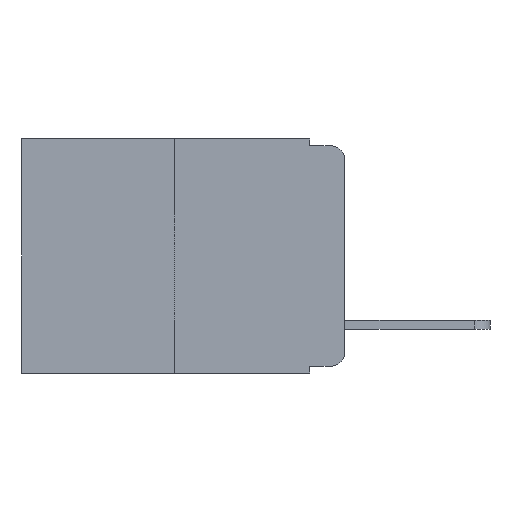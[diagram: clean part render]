
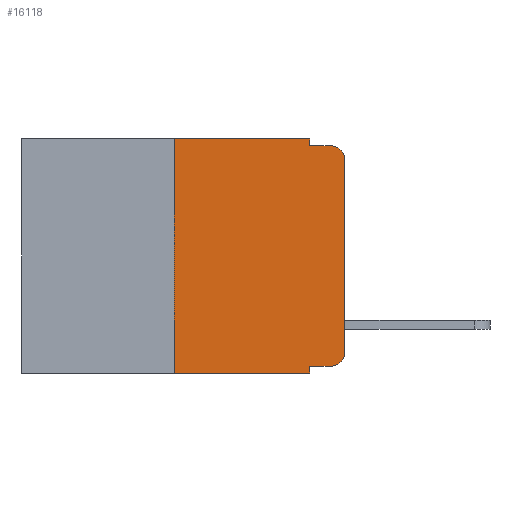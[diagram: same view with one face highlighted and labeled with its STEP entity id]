
A CAD part, left-side view. The second image highlights one B-rep face of the part: STEP entity #16118.
In plain terms, the highlighted planar face has unit normal (-1, 0, 0).
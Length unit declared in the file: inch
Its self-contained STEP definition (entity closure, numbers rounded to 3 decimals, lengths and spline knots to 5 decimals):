
#192 = ORIENTED_EDGE ( 'NONE', *, *, #7527, .T. ) ;
#748 = CARTESIAN_POINT ( 'NONE',  ( 0., 0.051, 0. ) ) ;
#917 = VERTEX_POINT ( 'NONE', #7803 ) ;
#1112 = CARTESIAN_POINT ( 'NONE',  ( 0., 0.02, -0.01 ) ) ;
#1442 = CARTESIAN_POINT ( 'NONE',  ( 0., 0.051, -0.343 ) ) ;
#1617 = DIRECTION ( 'NONE',  ( 0., 0., -1. ) ) ;
#1857 = ORIENTED_EDGE ( 'NONE', *, *, #20676, .T. ) ;
#2616 = CARTESIAN_POINT ( 'NONE',  ( 0., 0.25, 0. ) ) ;
#2884 = CIRCLE ( 'NONE', #18171, 0.02 ) ;
#3266 = DIRECTION ( 'NONE',  ( 0., 0., 1. ) ) ;
#3392 = VECTOR ( 'NONE', #4939, 39.37008 ) ;
#3632 = CARTESIAN_POINT ( 'NONE',  ( 0., 0.051, -0.01 ) ) ;
#3656 = DIRECTION ( 'NONE',  ( 0., 0., -1. ) ) ;
#3851 = DIRECTION ( 'NONE',  ( 0., 0., -1. ) ) ;
#3891 = DIRECTION ( 'NONE',  ( 0., 0., -1. ) ) ;
#3919 = VECTOR ( 'NONE', #3266, 39.37008 ) ;
#4071 = VECTOR ( 'NONE', #16908, 39.37008 ) ;
#4356 = LINE ( 'NONE', #11687, #6664 ) ;
#4586 = LINE ( 'NONE', #6137, #5873 ) ;
#4809 = CARTESIAN_POINT ( 'NONE',  ( 0., 0.02, -0.03 ) ) ;
#4848 = AXIS2_PLACEMENT_3D ( 'NONE', #6040, #10144, #3656 ) ;
#4939 = DIRECTION ( 'NONE',  ( 0., -1., 0. ) ) ;
#5044 = CIRCLE ( 'NONE', #7421, 0.02 ) ;
#5209 = CARTESIAN_POINT ( 'NONE',  ( 0., 0.473, -0.343 ) ) ;
#5281 = LINE ( 'NONE', #13376, #18626 ) ;
#5417 = LINE ( 'NONE', #15612, #9078 ) ;
#5488 = ORIENTED_EDGE ( 'NONE', *, *, #17545, .F. ) ;
#5578 = DIRECTION ( 'NONE',  ( -1., 0., 0. ) ) ;
#5608 = DIRECTION ( 'NONE',  ( 0., -1., 0. ) ) ;
#5873 = VECTOR ( 'NONE', #21460, 39.37008 ) ;
#6012 = LINE ( 'NONE', #6693, #3919 ) ;
#6040 = CARTESIAN_POINT ( 'NONE',  ( 0., 0.473, 0. ) ) ;
#6137 = CARTESIAN_POINT ( 'NONE',  ( 0., 0.25, 0. ) ) ;
#6664 = VECTOR ( 'NONE', #1617, 39.37008 ) ;
#6693 = CARTESIAN_POINT ( 'NONE',  ( 0., 0., 0. ) ) ;
#6850 = VERTEX_POINT ( 'NONE', #12879 ) ;
#7287 = CARTESIAN_POINT ( 'NONE',  ( 0., 0.25, -0.343 ) ) ;
#7421 = AXIS2_PLACEMENT_3D ( 'NONE', #4809, #9983, #11682 ) ;
#7527 = EDGE_CURVE ( 'NONE', #19859, #8125, #2884, .T. ) ;
#7785 = EDGE_CURVE ( 'NONE', #8125, #19622, #6012, .T. ) ;
#7803 = CARTESIAN_POINT ( 'NONE',  ( 0., 0.051, -0.333 ) ) ;
#7916 = EDGE_CURVE ( 'NONE', #18913, #11603, #14385, .T. ) ;
#8031 = VECTOR ( 'NONE', #3851, 39.37008 ) ;
#8125 = VERTEX_POINT ( 'NONE', #11254 ) ;
#8378 = ORIENTED_EDGE ( 'NONE', *, *, #7785, .T. ) ;
#8498 = LINE ( 'NONE', #5209, #4071 ) ;
#8711 = ORIENTED_EDGE ( 'NONE', *, *, #21223, .T. ) ;
#9006 = CARTESIAN_POINT ( 'NONE',  ( 0., 0.02, -0.313 ) ) ;
#9078 = VECTOR ( 'NONE', #5608, 39.37008 ) ;
#9328 = LINE ( 'NONE', #748, #8031 ) ;
#9983 = DIRECTION ( 'NONE',  ( -1., 0., 0. ) ) ;
#10144 = DIRECTION ( 'NONE',  ( 1., 0., 0. ) ) ;
#10341 = CARTESIAN_POINT ( 'NONE',  ( 0., 0.02, -0.333 ) ) ;
#11108 = CARTESIAN_POINT ( 'NONE',  ( 0., 0., -0.03 ) ) ;
#11205 = VERTEX_POINT ( 'NONE', #1442 ) ;
#11254 = CARTESIAN_POINT ( 'NONE',  ( 0., 0., -0.313 ) ) ;
#11603 = VERTEX_POINT ( 'NONE', #1112 ) ;
#11682 = DIRECTION ( 'NONE',  ( 0., 0., -1. ) ) ;
#11687 = CARTESIAN_POINT ( 'NONE',  ( 0., 0.051, 0. ) ) ;
#12037 = ORIENTED_EDGE ( 'NONE', *, *, #15111, .T. ) ;
#12457 = EDGE_LOOP ( 'NONE', ( #8378, #8711, #18246, #17860, #18544, #5488, #12037, #12544, #1857, #192 ) ) ;
#12458 = VERTEX_POINT ( 'NONE', #2616 ) ;
#12544 = ORIENTED_EDGE ( 'NONE', *, *, #16888, .F. ) ;
#12879 = CARTESIAN_POINT ( 'NONE',  ( 0., 0.051, 0. ) ) ;
#12886 = CARTESIAN_POINT ( 'NONE',  ( 0., 0.051, -0.01 ) ) ;
#13376 = CARTESIAN_POINT ( 'NONE',  ( 0., 0.051, -0.333 ) ) ;
#14385 = LINE ( 'NONE', #3632, #3392 ) ;
#15111 = EDGE_CURVE ( 'NONE', #16461, #11205, #8498, .T. ) ;
#15612 = CARTESIAN_POINT ( 'NONE',  ( 0., 0.473, 0. ) ) ;
#15962 = EDGE_CURVE ( 'NONE', #12458, #6850, #5417, .T. ) ;
#15994 = EDGE_CURVE ( 'NONE', #6850, #18913, #9328, .T. ) ;
#16118 = ADVANCED_FACE ( 'NONE', ( #21424 ), #19380, .F. ) ;
#16461 = VERTEX_POINT ( 'NONE', #7287 ) ;
#16888 = EDGE_CURVE ( 'NONE', #917, #11205, #4356, .T. ) ;
#16908 = DIRECTION ( 'NONE',  ( 0., -1., 0. ) ) ;
#17026 = DIRECTION ( 'NONE',  ( 0., -1., 0. ) ) ;
#17545 = EDGE_CURVE ( 'NONE', #16461, #12458, #4586, .T. ) ;
#17860 = ORIENTED_EDGE ( 'NONE', *, *, #15994, .F. ) ;
#18171 = AXIS2_PLACEMENT_3D ( 'NONE', #9006, #5578, #3891 ) ;
#18246 = ORIENTED_EDGE ( 'NONE', *, *, #7916, .F. ) ;
#18544 = ORIENTED_EDGE ( 'NONE', *, *, #15962, .F. ) ;
#18626 = VECTOR ( 'NONE', #17026, 39.37008 ) ;
#18913 = VERTEX_POINT ( 'NONE', #12886 ) ;
#19380 = PLANE ( 'NONE',  #4848 ) ;
#19622 = VERTEX_POINT ( 'NONE', #11108 ) ;
#19859 = VERTEX_POINT ( 'NONE', #10341 ) ;
#20676 = EDGE_CURVE ( 'NONE', #917, #19859, #5281, .T. ) ;
#21223 = EDGE_CURVE ( 'NONE', #19622, #11603, #5044, .T. ) ;
#21424 = FACE_OUTER_BOUND ( 'NONE', #12457, .T. ) ;
#21460 = DIRECTION ( 'NONE',  ( 0., 0., 1. ) ) ;
